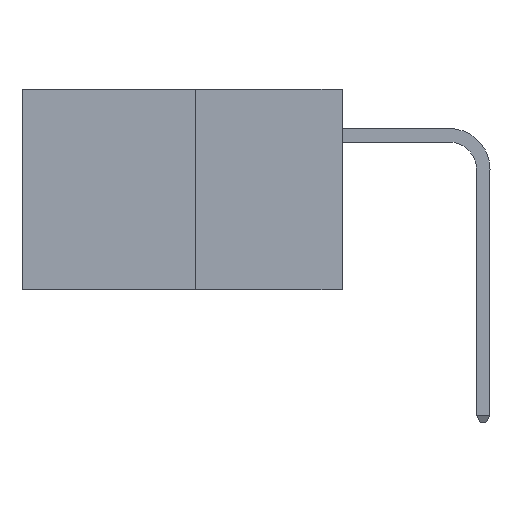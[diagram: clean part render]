
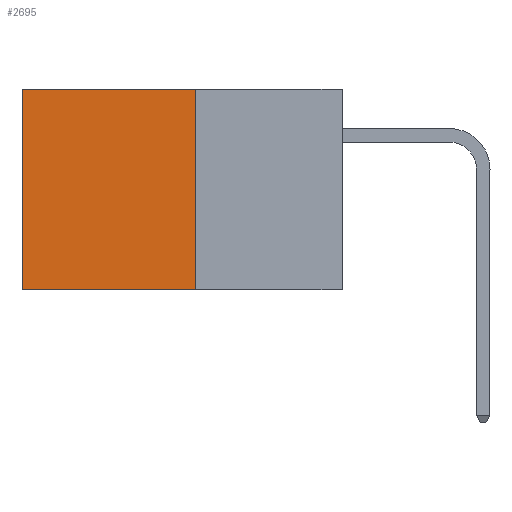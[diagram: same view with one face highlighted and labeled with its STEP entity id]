
A CAD part, left-side view. The second image highlights one B-rep face of the part: STEP entity #2695.
In plain terms, the highlighted planar face has unit normal (-1, 0, 0).
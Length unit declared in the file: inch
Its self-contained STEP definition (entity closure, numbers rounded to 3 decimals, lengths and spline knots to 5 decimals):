
#34 = LINE ( 'NONE', #5961, #10772 ) ;
#56 = AXIS2_PLACEMENT_3D ( 'NONE', #9607, #8229, #8056 ) ;
#389 = VERTEX_POINT ( 'NONE', #10954 ) ;
#850 = VECTOR ( 'NONE', #2992, 39.37008 ) ;
#2464 = CARTESIAN_POINT ( 'NONE',  ( 0.277, 0.59, 0. ) ) ;
#2695 = ADVANCED_FACE ( 'NONE', ( #10144 ), #8847, .F. ) ;
#2992 = DIRECTION ( 'NONE',  ( 0., 1., 0. ) ) ;
#3010 = ORIENTED_EDGE ( 'NONE', *, *, #9439, .T. ) ;
#3344 = ORIENTED_EDGE ( 'NONE', *, *, #8097, .F. ) ;
#3688 = ORIENTED_EDGE ( 'NONE', *, *, #13196, .T. ) ;
#4034 = VERTEX_POINT ( 'NONE', #10007 ) ;
#4124 = DIRECTION ( 'NONE',  ( 0., 1., 0. ) ) ;
#5961 = CARTESIAN_POINT ( 'NONE',  ( 0.277, 0.27, -0.37 ) ) ;
#7730 = LINE ( 'NONE', #10202, #13050 ) ;
#8009 = DIRECTION ( 'NONE',  ( 0., 0., -1. ) ) ;
#8056 = DIRECTION ( 'NONE',  ( 0., 0., -1. ) ) ;
#8097 = EDGE_CURVE ( 'NONE', #389, #4034, #34, .T. ) ;
#8229 = DIRECTION ( 'NONE',  ( 1., 0., 0. ) ) ;
#8683 = CARTESIAN_POINT ( 'NONE',  ( 0.277, 0.59, -0.37 ) ) ;
#8847 = PLANE ( 'NONE',  #56 ) ;
#8948 = EDGE_LOOP ( 'NONE', ( #3010, #11179, #3344, #3688 ) ) ;
#9439 = EDGE_CURVE ( 'NONE', #10662, #10088, #12523, .T. ) ;
#9469 = LINE ( 'NONE', #13062, #850 ) ;
#9607 = CARTESIAN_POINT ( 'NONE',  ( 0.277, 0.27, -0.37 ) ) ;
#10007 = CARTESIAN_POINT ( 'NONE',  ( 0.277, 0.27, -0.37 ) ) ;
#10088 = VERTEX_POINT ( 'NONE', #11975 ) ;
#10144 = FACE_OUTER_BOUND ( 'NONE', #8948, .T. ) ;
#10185 = VECTOR ( 'NONE', #10730, 39.37008 ) ;
#10202 = CARTESIAN_POINT ( 'NONE',  ( 0.277, 0.27, -0.37 ) ) ;
#10662 = VERTEX_POINT ( 'NONE', #2464 ) ;
#10730 = DIRECTION ( 'NONE',  ( 0., 0., -1. ) ) ;
#10772 = VECTOR ( 'NONE', #8009, 39.37008 ) ;
#10954 = CARTESIAN_POINT ( 'NONE',  ( 0.277, 0.27, 0. ) ) ;
#11179 = ORIENTED_EDGE ( 'NONE', *, *, #13058, .F. ) ;
#11975 = CARTESIAN_POINT ( 'NONE',  ( 0.277, 0.59, -0.37 ) ) ;
#12523 = LINE ( 'NONE', #8683, #10185 ) ;
#13050 = VECTOR ( 'NONE', #4124, 39.37008 ) ;
#13058 = EDGE_CURVE ( 'NONE', #4034, #10088, #7730, .T. ) ;
#13062 = CARTESIAN_POINT ( 'NONE',  ( 0.277, 0.27, 0. ) ) ;
#13196 = EDGE_CURVE ( 'NONE', #389, #10662, #9469, .T. ) ;
